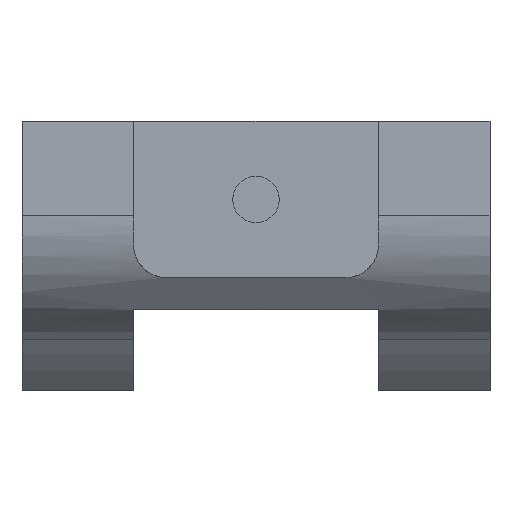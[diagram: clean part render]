
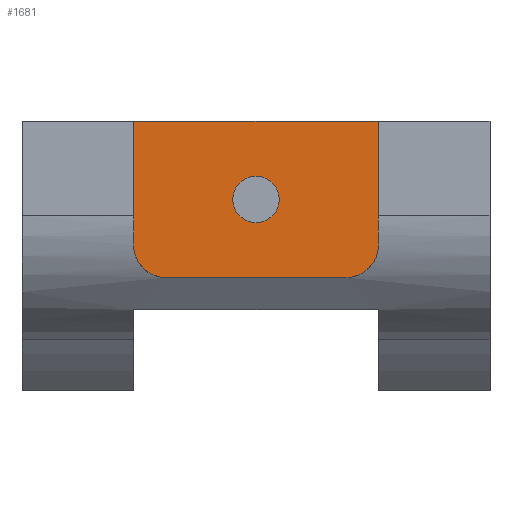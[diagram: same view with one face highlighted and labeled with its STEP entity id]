
A CAD part, front view. The second image highlights one B-rep face of the part: STEP entity #1681.
In plain terms, the highlighted planar face has unit normal (0, -1, 0).
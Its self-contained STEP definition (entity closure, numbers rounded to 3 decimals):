
#49 = ORIENTED_EDGE ( 'NONE', *, *, #497, .F. ) ;
#69 = VECTOR ( 'NONE', #234, 1000. ) ;
#78 = DIRECTION ( 'NONE',  ( 1., 0., 0. ) ) ;
#122 = CARTESIAN_POINT ( 'NONE',  ( 4.381, 3.175, -7.62 ) ) ;
#123 = EDGE_CURVE ( 'NONE', #2132, #1184, #1785, .T. ) ;
#153 = ORIENTED_EDGE ( 'NONE', *, *, #2091, .F. ) ;
#183 = CARTESIAN_POINT ( 'NONE',  ( 0., 3.175, -3.81 ) ) ;
#234 = DIRECTION ( 'NONE',  ( 0., 0., -1. ) ) ;
#239 = ORIENTED_EDGE ( 'NONE', *, *, #1177, .T. ) ;
#243 = ORIENTED_EDGE ( 'NONE', *, *, #433, .T. ) ;
#251 = VERTEX_POINT ( 'NONE', #122 ) ;
#300 = CIRCLE ( 'NONE', #1837, 1.588 ) ;
#368 = DIRECTION ( 'NONE',  ( 0., 0., -1. ) ) ;
#376 = CARTESIAN_POINT ( 'NONE',  ( 5.969, 3.175, 0. ) ) ;
#426 = CARTESIAN_POINT ( 'NONE',  ( 0., 3.175, -2.68 ) ) ;
#433 = EDGE_CURVE ( 'NONE', #1039, #2265, #1547, .T. ) ;
#474 = VERTEX_POINT ( 'NONE', #1794 ) ;
#497 = EDGE_CURVE ( 'NONE', #1184, #2132, #2336, .T. ) ;
#498 = CARTESIAN_POINT ( 'NONE',  ( 5.969, 3.175, 0. ) ) ;
#538 = VERTEX_POINT ( 'NONE', #1989 ) ;
#602 = DIRECTION ( 'NONE',  ( 0., -1., 0. ) ) ;
#606 = EDGE_LOOP ( 'NONE', ( #2170, #49 ) ) ;
#626 = EDGE_CURVE ( 'NONE', #251, #474, #300, .T. ) ;
#665 = EDGE_CURVE ( 'NONE', #1612, #251, #2305, .T. ) ;
#686 = DIRECTION ( 'NONE',  ( 0., 0., -1. ) ) ;
#692 = CARTESIAN_POINT ( 'NONE',  ( 0., 3.175, -4.94 ) ) ;
#694 = DIRECTION ( 'NONE',  ( 0., -1., 0. ) ) ;
#707 = VECTOR ( 'NONE', #686, 1000. ) ;
#712 = DIRECTION ( 'NONE',  ( -1., 0., 0. ) ) ;
#731 = ORIENTED_EDGE ( 'NONE', *, *, #665, .T. ) ;
#787 = DIRECTION ( 'NONE',  ( 0., 0., -1. ) ) ;
#799 = CARTESIAN_POINT ( 'NONE',  ( 0., 3.175, -7.62 ) ) ;
#869 = CARTESIAN_POINT ( 'NONE',  ( -4.381, 3.175, -6.032 ) ) ;
#885 = AXIS2_PLACEMENT_3D ( 'NONE', #183, #1454, #368 ) ;
#937 = DIRECTION ( 'NONE',  ( 0., -1., 0. ) ) ;
#947 = CARTESIAN_POINT ( 'NONE',  ( 0., 3.175, -3.81 ) ) ;
#970 = FACE_OUTER_BOUND ( 'NONE', #1218, .T. ) ;
#1039 = VERTEX_POINT ( 'NONE', #376 ) ;
#1053 = DIRECTION ( 'NONE',  ( 0., 0., -1. ) ) ;
#1091 = LINE ( 'NONE', #1142, #69 ) ;
#1142 = CARTESIAN_POINT ( 'NONE',  ( -5.969, 3.175, 0. ) ) ;
#1177 = EDGE_CURVE ( 'NONE', #2265, #538, #1091, .T. ) ;
#1184 = VERTEX_POINT ( 'NONE', #426 ) ;
#1218 = EDGE_LOOP ( 'NONE', ( #239, #1623, #731, #1939, #153, #243 ) ) ;
#1224 = AXIS2_PLACEMENT_3D ( 'NONE', #869, #2117, #1053 ) ;
#1261 = CARTESIAN_POINT ( 'NONE',  ( 0., 3.175, 0. ) ) ;
#1407 = PLANE ( 'NONE',  #2294 ) ;
#1415 = CARTESIAN_POINT ( 'NONE',  ( 0., 3.175, 0. ) ) ;
#1454 = DIRECTION ( 'NONE',  ( 0., -1., 0. ) ) ;
#1456 = FACE_BOUND ( 'NONE', #606, .T. ) ;
#1547 = LINE ( 'NONE', #1261, #1974 ) ;
#1553 = CARTESIAN_POINT ( 'NONE',  ( -4.381, 3.175, -7.62 ) ) ;
#1612 = VERTEX_POINT ( 'NONE', #1553 ) ;
#1623 = ORIENTED_EDGE ( 'NONE', *, *, #1664, .T. ) ;
#1664 = EDGE_CURVE ( 'NONE', #538, #1612, #2040, .T. ) ;
#1665 = LINE ( 'NONE', #498, #707 ) ;
#1681 = ADVANCED_FACE ( 'NONE', ( #1456, #970 ), #1407, .T. ) ;
#1686 = CARTESIAN_POINT ( 'NONE',  ( 4.381, 3.175, -6.032 ) ) ;
#1695 = AXIS2_PLACEMENT_3D ( 'NONE', #947, #937, #787 ) ;
#1785 = CIRCLE ( 'NONE', #1695, 1.13 ) ;
#1794 = CARTESIAN_POINT ( 'NONE',  ( 5.969, 3.175, -6.032 ) ) ;
#1826 = VECTOR ( 'NONE', #78, 1000. ) ;
#1837 = AXIS2_PLACEMENT_3D ( 'NONE', #1686, #602, #1863 ) ;
#1863 = DIRECTION ( 'NONE',  ( 0., 0., -1. ) ) ;
#1939 = ORIENTED_EDGE ( 'NONE', *, *, #626, .T. ) ;
#1950 = DIRECTION ( 'NONE',  ( 0., 0., -1. ) ) ;
#1974 = VECTOR ( 'NONE', #712, 1000. ) ;
#1989 = CARTESIAN_POINT ( 'NONE',  ( -5.969, 3.175, -6.032 ) ) ;
#2040 = CIRCLE ( 'NONE', #1224, 1.588 ) ;
#2085 = CARTESIAN_POINT ( 'NONE',  ( -5.969, 3.175, 0. ) ) ;
#2091 = EDGE_CURVE ( 'NONE', #1039, #474, #1665, .T. ) ;
#2117 = DIRECTION ( 'NONE',  ( 0., -1., 0. ) ) ;
#2132 = VERTEX_POINT ( 'NONE', #692 ) ;
#2170 = ORIENTED_EDGE ( 'NONE', *, *, #123, .F. ) ;
#2265 = VERTEX_POINT ( 'NONE', #2085 ) ;
#2294 = AXIS2_PLACEMENT_3D ( 'NONE', #1415, #694, #1950 ) ;
#2305 = LINE ( 'NONE', #799, #1826 ) ;
#2336 = CIRCLE ( 'NONE', #885, 1.13 ) ;
